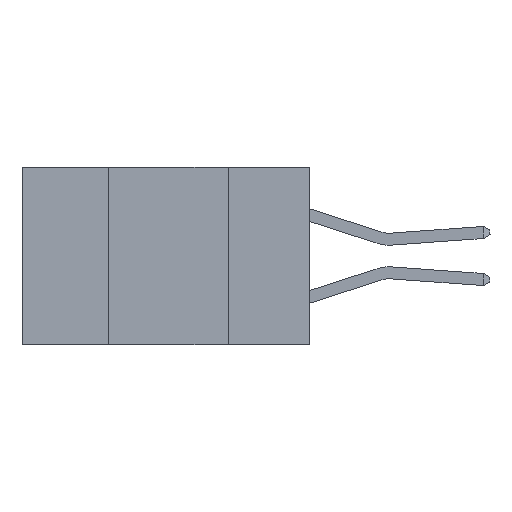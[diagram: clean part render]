
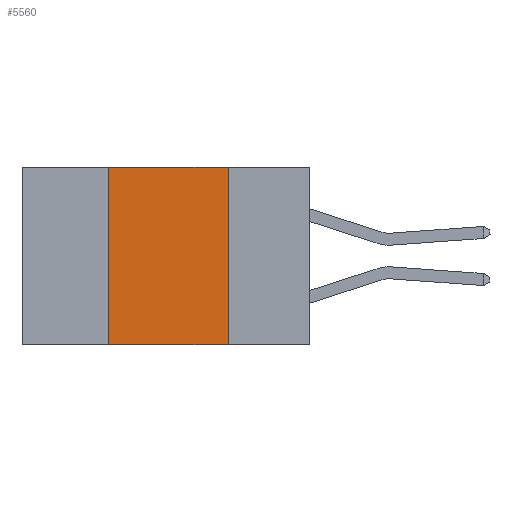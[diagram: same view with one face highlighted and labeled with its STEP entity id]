
A CAD part, left-side view. The second image highlights one B-rep face of the part: STEP entity #5560.
In plain terms, the highlighted planar face has unit normal (-1, 0, 0).
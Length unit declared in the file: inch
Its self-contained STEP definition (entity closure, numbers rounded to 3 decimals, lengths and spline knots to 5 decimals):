
#1255 = VERTEX_POINT ( 'NONE', #20642 ) ;
#1398 = VERTEX_POINT ( 'NONE', #10290 ) ;
#2760 = VECTOR ( 'NONE', #19319, 39.37008 ) ;
#5297 = VECTOR ( 'NONE', #5486, 39.37008 ) ;
#5408 = CARTESIAN_POINT ( 'NONE',  ( 0., 0.6, 0. ) ) ;
#5470 = EDGE_CURVE ( 'NONE', #1398, #19044, #21136, .T. ) ;
#5486 = DIRECTION ( 'NONE',  ( 0., 0., -1. ) ) ;
#5560 = ADVANCED_FACE ( 'NONE', ( #13922 ), #5841, .F. ) ;
#5841 = PLANE ( 'NONE',  #7514 ) ;
#7514 = AXIS2_PLACEMENT_3D ( 'NONE', #5408, #11291, #12662 ) ;
#7734 = CARTESIAN_POINT ( 'NONE',  ( 0., 0.17, 0. ) ) ;
#7949 = ORIENTED_EDGE ( 'NONE', *, *, #5470, .F. ) ;
#8075 = CARTESIAN_POINT ( 'NONE',  ( 0., 0.6, -0.37 ) ) ;
#9516 = CARTESIAN_POINT ( 'NONE',  ( 0., 0.42, 0. ) ) ;
#10290 = CARTESIAN_POINT ( 'NONE',  ( 0., 0.42, -0.37 ) ) ;
#11291 = DIRECTION ( 'NONE',  ( 1., 0., 0. ) ) ;
#11432 = EDGE_CURVE ( 'NONE', #1255, #26763, #22806, .T. ) ;
#12041 = EDGE_LOOP ( 'NONE', ( #15705, #21359, #7949, #17162 ) ) ;
#12662 = DIRECTION ( 'NONE',  ( 0., 0., -1. ) ) ;
#13922 = FACE_OUTER_BOUND ( 'NONE', #12041, .T. ) ;
#15300 = VECTOR ( 'NONE', #26179, 39.37008 ) ;
#15705 = ORIENTED_EDGE ( 'NONE', *, *, #11432, .F. ) ;
#17101 = CARTESIAN_POINT ( 'NONE',  ( 0., 0.6, 0. ) ) ;
#17162 = ORIENTED_EDGE ( 'NONE', *, *, #27891, .T. ) ;
#17342 = LINE ( 'NONE', #8075, #28071 ) ;
#17729 = CARTESIAN_POINT ( 'NONE',  ( 0., 0.17, -0.37 ) ) ;
#19044 = VERTEX_POINT ( 'NONE', #20117 ) ;
#19045 = DIRECTION ( 'NONE',  ( 0., -1., 0. ) ) ;
#19319 = DIRECTION ( 'NONE',  ( 0., -1., 0. ) ) ;
#20117 = CARTESIAN_POINT ( 'NONE',  ( 0., 0.42, 0. ) ) ;
#20377 = LINE ( 'NONE', #17101, #2760 ) ;
#20642 = CARTESIAN_POINT ( 'NONE',  ( 0., 0.17, 0. ) ) ;
#21136 = LINE ( 'NONE', #9516, #15300 ) ;
#21359 = ORIENTED_EDGE ( 'NONE', *, *, #21897, .F. ) ;
#21897 = EDGE_CURVE ( 'NONE', #19044, #1255, #20377, .T. ) ;
#22806 = LINE ( 'NONE', #7734, #5297 ) ;
#26179 = DIRECTION ( 'NONE',  ( 0., 0., 1. ) ) ;
#26763 = VERTEX_POINT ( 'NONE', #17729 ) ;
#27891 = EDGE_CURVE ( 'NONE', #1398, #26763, #17342, .T. ) ;
#28071 = VECTOR ( 'NONE', #19045, 39.37008 ) ;
